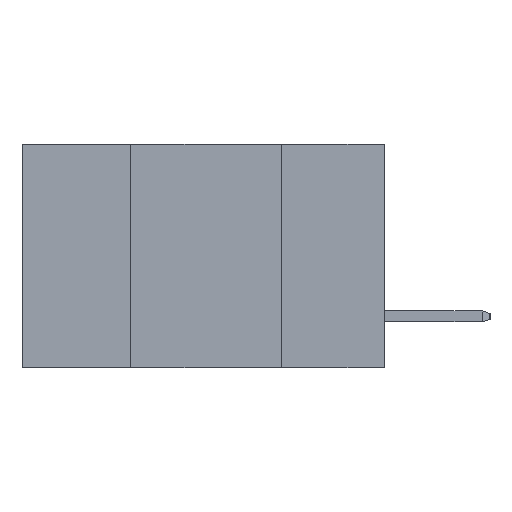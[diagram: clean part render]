
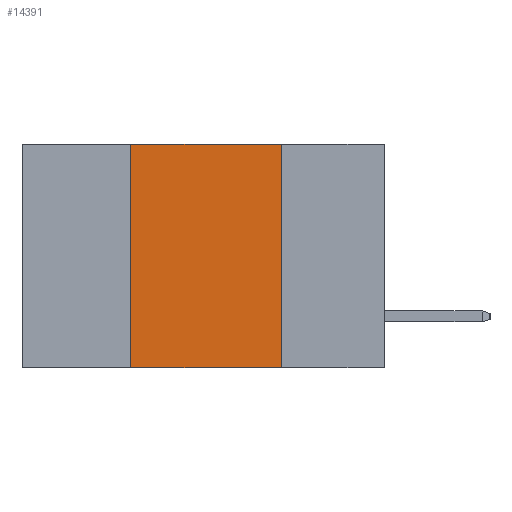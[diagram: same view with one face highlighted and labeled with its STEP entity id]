
A CAD part, left-side view. The second image highlights one B-rep face of the part: STEP entity #14391.
In plain terms, the highlighted planar face has unit normal (-1, 0, 0).
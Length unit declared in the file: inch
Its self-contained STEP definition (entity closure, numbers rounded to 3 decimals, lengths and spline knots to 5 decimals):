
#94 = DIRECTION ( 'NONE',  ( 1., 0., 0. ) ) ;
#297 = CARTESIAN_POINT ( 'NONE',  ( 0., 0.6, -0.37 ) ) ;
#954 = LINE ( 'NONE', #14479, #12751 ) ;
#1057 = LINE ( 'NONE', #297, #8427 ) ;
#1720 = VERTEX_POINT ( 'NONE', #6905 ) ;
#2727 = LINE ( 'NONE', #15426, #13993 ) ;
#3771 = ORIENTED_EDGE ( 'NONE', *, *, #18287, .F. ) ;
#5154 = DIRECTION ( 'NONE',  ( 0., 0., 1. ) ) ;
#5589 = ORIENTED_EDGE ( 'NONE', *, *, #13584, .F. ) ;
#6027 = LINE ( 'NONE', #15425, #17182 ) ;
#6182 = VERTEX_POINT ( 'NONE', #17352 ) ;
#6905 = CARTESIAN_POINT ( 'NONE',  ( 0., 0.42, 0. ) ) ;
#7473 = CARTESIAN_POINT ( 'NONE',  ( 0., 0.6, 0. ) ) ;
#7937 = CARTESIAN_POINT ( 'NONE',  ( 0., 0.17, -0.37 ) ) ;
#8022 = DIRECTION ( 'NONE',  ( 0., 0., -1. ) ) ;
#8427 = VECTOR ( 'NONE', #9150, 39.37008 ) ;
#8604 = DIRECTION ( 'NONE',  ( 0., -1., 0. ) ) ;
#9073 = CARTESIAN_POINT ( 'NONE',  ( 0., 0.42, -0.37 ) ) ;
#9150 = DIRECTION ( 'NONE',  ( 0., -1., 0. ) ) ;
#10374 = FACE_OUTER_BOUND ( 'NONE', #17258, .T. ) ;
#10380 = PLANE ( 'NONE',  #10449 ) ;
#10439 = DIRECTION ( 'NONE',  ( 0., 0., -1. ) ) ;
#10449 = AXIS2_PLACEMENT_3D ( 'NONE', #7473, #94, #10439 ) ;
#10578 = EDGE_CURVE ( 'NONE', #16416, #15908, #1057, .T. ) ;
#12516 = ORIENTED_EDGE ( 'NONE', *, *, #15515, .F. ) ;
#12751 = VECTOR ( 'NONE', #8604, 39.37008 ) ;
#13584 = EDGE_CURVE ( 'NONE', #16416, #1720, #6027, .T. ) ;
#13993 = VECTOR ( 'NONE', #8022, 39.37008 ) ;
#14359 = ORIENTED_EDGE ( 'NONE', *, *, #10578, .T. ) ;
#14391 = ADVANCED_FACE ( 'NONE', ( #10374 ), #10380, .F. ) ;
#14479 = CARTESIAN_POINT ( 'NONE',  ( 0., 0.6, 0. ) ) ;
#15425 = CARTESIAN_POINT ( 'NONE',  ( 0., 0.42, -0.37 ) ) ;
#15426 = CARTESIAN_POINT ( 'NONE',  ( 0., 0.17, -0.37 ) ) ;
#15515 = EDGE_CURVE ( 'NONE', #1720, #6182, #954, .T. ) ;
#15908 = VERTEX_POINT ( 'NONE', #7937 ) ;
#16416 = VERTEX_POINT ( 'NONE', #9073 ) ;
#17182 = VECTOR ( 'NONE', #5154, 39.37008 ) ;
#17258 = EDGE_LOOP ( 'NONE', ( #3771, #12516, #5589, #14359 ) ) ;
#17352 = CARTESIAN_POINT ( 'NONE',  ( 0., 0.17, 0. ) ) ;
#18287 = EDGE_CURVE ( 'NONE', #6182, #15908, #2727, .T. ) ;
